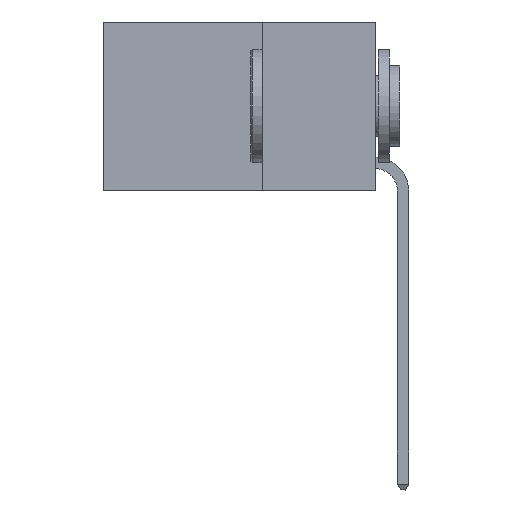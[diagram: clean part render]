
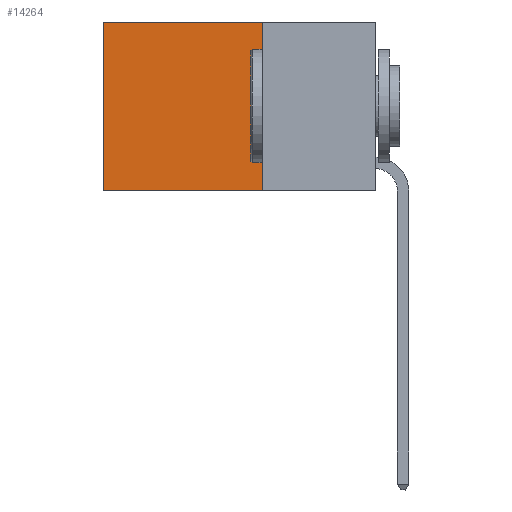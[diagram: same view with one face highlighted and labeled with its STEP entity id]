
A CAD part, left-side view. The second image highlights one B-rep face of the part: STEP entity #14264.
In plain terms, the highlighted planar face has unit normal (-1, 0, 0).
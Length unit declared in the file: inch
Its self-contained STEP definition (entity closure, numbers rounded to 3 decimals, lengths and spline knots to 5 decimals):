
#1400 = DIRECTION ( 'NONE',  ( 0., 0., -1. ) ) ;
#1740 = VERTEX_POINT ( 'NONE', #17830 ) ;
#3348 = VERTEX_POINT ( 'NONE', #16308 ) ;
#3777 = LINE ( 'NONE', #18350, #17433 ) ;
#3846 = DIRECTION ( 'NONE',  ( 0., 1., 0. ) ) ;
#4036 = CARTESIAN_POINT ( 'NONE',  ( 0.2625, 0.6, 0. ) ) ;
#5773 = DIRECTION ( 'NONE',  ( 0., 0., -1. ) ) ;
#6344 = CARTESIAN_POINT ( 'NONE',  ( 0.2625, 0.25, 0. ) ) ;
#8223 = LINE ( 'NONE', #25086, #19525 ) ;
#8242 = DIRECTION ( 'NONE',  ( 1., 0., 0. ) ) ;
#8496 = ORIENTED_EDGE ( 'NONE', *, *, #18510, .T. ) ;
#10411 = VECTOR ( 'NONE', #3846, 39.37008 ) ;
#10627 = ORIENTED_EDGE ( 'NONE', *, *, #22298, .T. ) ;
#10628 = LINE ( 'NONE', #6344, #25656 ) ;
#11910 = VERTEX_POINT ( 'NONE', #4036 ) ;
#12157 = DIRECTION ( 'NONE',  ( 0., 1., 0. ) ) ;
#12252 = FACE_OUTER_BOUND ( 'NONE', #16902, .T. ) ;
#12614 = EDGE_CURVE ( 'NONE', #3348, #1740, #10628, .T. ) ;
#14264 = ADVANCED_FACE ( 'NONE', ( #12252 ), #18445, .F. ) ;
#14288 = LINE ( 'NONE', #22720, #10411 ) ;
#14315 = CARTESIAN_POINT ( 'NONE',  ( 0.2625, 0.25, 0. ) ) ;
#14757 = DIRECTION ( 'NONE',  ( 0., 0., -1. ) ) ;
#16308 = CARTESIAN_POINT ( 'NONE',  ( 0.2625, 0.25, 0. ) ) ;
#16902 = EDGE_LOOP ( 'NONE', ( #8496, #19758, #21261, #10627 ) ) ;
#17433 = VECTOR ( 'NONE', #12157, 39.37008 ) ;
#17830 = CARTESIAN_POINT ( 'NONE',  ( 0.2625, 0.25, -0.37 ) ) ;
#18350 = CARTESIAN_POINT ( 'NONE',  ( 0.2625, 0.25, 0. ) ) ;
#18445 = PLANE ( 'NONE',  #26820 ) ;
#18510 = EDGE_CURVE ( 'NONE', #11910, #22534, #8223, .T. ) ;
#19525 = VECTOR ( 'NONE', #1400, 39.37008 ) ;
#19758 = ORIENTED_EDGE ( 'NONE', *, *, #22521, .F. ) ;
#20502 = CARTESIAN_POINT ( 'NONE',  ( 0.2625, 0.6, -0.37 ) ) ;
#21261 = ORIENTED_EDGE ( 'NONE', *, *, #12614, .F. ) ;
#22298 = EDGE_CURVE ( 'NONE', #3348, #11910, #3777, .T. ) ;
#22521 = EDGE_CURVE ( 'NONE', #1740, #22534, #14288, .T. ) ;
#22534 = VERTEX_POINT ( 'NONE', #20502 ) ;
#22720 = CARTESIAN_POINT ( 'NONE',  ( 0.2625, 0.25, -0.37 ) ) ;
#25086 = CARTESIAN_POINT ( 'NONE',  ( 0.2625, 0.6, 0. ) ) ;
#25656 = VECTOR ( 'NONE', #14757, 39.37008 ) ;
#26820 = AXIS2_PLACEMENT_3D ( 'NONE', #14315, #8242, #5773 ) ;
